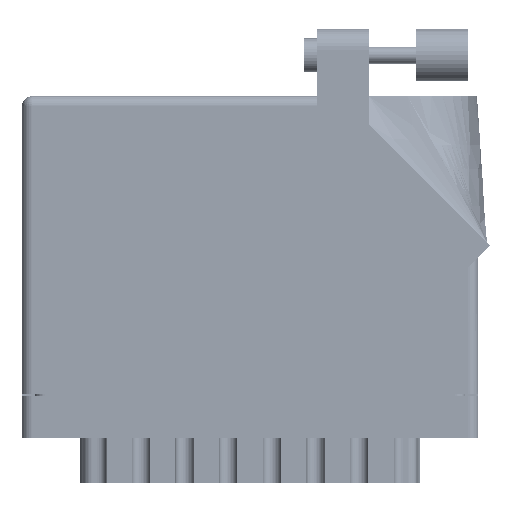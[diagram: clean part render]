
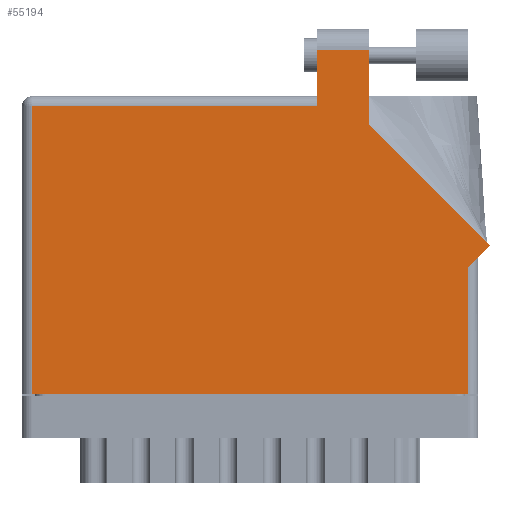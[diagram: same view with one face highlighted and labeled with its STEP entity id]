
A CAD part, front view. The second image highlights one B-rep face of the part: STEP entity #55194.
In plain terms, the highlighted face is planar.
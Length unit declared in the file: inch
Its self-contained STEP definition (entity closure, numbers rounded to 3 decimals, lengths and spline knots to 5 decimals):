
#117 = VECTOR ( 'NONE', #33223, 39.37008 ) ;
#1167 = VERTEX_POINT ( 'NONE', #13531 ) ;
#1967 = LINE ( 'NONE', #8694, #117 ) ;
#3951 = ORIENTED_EDGE ( 'NONE', *, *, #8646, .T. ) ;
#4940 = EDGE_CURVE ( 'NONE', #1167, #25497, #57573, .T. ) ;
#6909 = PLANE ( 'NONE',  #57899 ) ;
#6983 = CARTESIAN_POINT ( 'NONE',  ( 0.062, 1.713, 0. ) ) ;
#8646 = EDGE_CURVE ( 'NONE', #9495, #41288, #15543, .T. ) ;
#8694 = CARTESIAN_POINT ( 'NONE',  ( 1.758, 1.775, 0. ) ) ;
#9495 = VERTEX_POINT ( 'NONE', #6983 ) ;
#10951 = LINE ( 'NONE', #35171, #68198 ) ;
#11305 = ORIENTED_EDGE ( 'NONE', *, *, #34914, .T. ) ;
#13531 = CARTESIAN_POINT ( 'NONE',  ( 2.78871, 0.88571, 0. ) ) ;
#13729 = VECTOR ( 'NONE', #26356, 39.37008 ) ;
#13963 = EDGE_CURVE ( 'NONE', #33533, #1167, #19440, .T. ) ;
#14648 = CARTESIAN_POINT ( 'NONE',  ( 2.656, 0.815, 0. ) ) ;
#15543 = LINE ( 'NONE', #58192, #41485 ) ;
#16351 = DIRECTION ( 'NONE',  ( 0.707, 0.707, 0. ) ) ;
#17807 = DIRECTION ( 'NONE',  ( 1., 0., 0. ) ) ;
#18433 = CARTESIAN_POINT ( 'NONE',  ( 0., 1.713, 0. ) ) ;
#19440 = LINE ( 'NONE', #59026, #32470 ) ;
#19483 = CARTESIAN_POINT ( 'NONE',  ( 0., 1.775, 0. ) ) ;
#21790 = DIRECTION ( 'NONE',  ( 0., 1., 0. ) ) ;
#23983 = VECTOR ( 'NONE', #42228, 39.37008 ) ;
#25497 = VERTEX_POINT ( 'NONE', #66298 ) ;
#26232 = FACE_OUTER_BOUND ( 'NONE', #36542, .T. ) ;
#26356 = DIRECTION ( 'NONE',  ( 0., 1., 0. ) ) ;
#26746 = LINE ( 'NONE', #14648, #13729 ) ;
#29104 = CARTESIAN_POINT ( 'NONE',  ( 1.758, 1.713, 0. ) ) ;
#29597 = EDGE_CURVE ( 'NONE', #49752, #9495, #55372, .T. ) ;
#30723 = LINE ( 'NONE', #57432, #52042 ) ;
#31455 = CARTESIAN_POINT ( 'NONE',  ( 2.656, 0.753, 0. ) ) ;
#31815 = ORIENTED_EDGE ( 'NONE', *, *, #45320, .T. ) ;
#32470 = VECTOR ( 'NONE', #16351, 39.37008 ) ;
#32636 = VECTOR ( 'NONE', #74051, 39.37008 ) ;
#33223 = DIRECTION ( 'NONE',  ( 0., -1., 0. ) ) ;
#33486 = LINE ( 'NONE', #73520, #64881 ) ;
#33533 = VERTEX_POINT ( 'NONE', #31455 ) ;
#34914 = EDGE_CURVE ( 'NONE', #44248, #49752, #1967, .T. ) ;
#35171 = CARTESIAN_POINT ( 'NONE',  ( 0., 0., 0. ) ) ;
#36542 = EDGE_LOOP ( 'NONE', ( #62070, #53210, #11305, #51269, #3951, #51979, #31815, #52541, #62905 ) ) ;
#39656 = EDGE_CURVE ( 'NONE', #41288, #51704, #10951, .T. ) ;
#40179 = CARTESIAN_POINT ( 'NONE',  ( 1.758, 2.05, 0. ) ) ;
#40978 = DIRECTION ( 'NONE',  ( 0., 0., -1. ) ) ;
#41288 = VERTEX_POINT ( 'NONE', #68740 ) ;
#41485 = VECTOR ( 'NONE', #70073, 39.37008 ) ;
#42228 = DIRECTION ( 'NONE',  ( -1., 0., 0. ) ) ;
#44248 = VERTEX_POINT ( 'NONE', #40179 ) ;
#45320 = EDGE_CURVE ( 'NONE', #51704, #33533, #26746, .T. ) ;
#48460 = DIRECTION ( 'NONE',  ( -1., 0., 0. ) ) ;
#49752 = VERTEX_POINT ( 'NONE', #29104 ) ;
#51269 = ORIENTED_EDGE ( 'NONE', *, *, #29597, .T. ) ;
#51704 = VERTEX_POINT ( 'NONE', #68649 ) ;
#51979 = ORIENTED_EDGE ( 'NONE', *, *, #39656, .T. ) ;
#52042 = VECTOR ( 'NONE', #21790, 39.37008 ) ;
#52541 = ORIENTED_EDGE ( 'NONE', *, *, #13963, .T. ) ;
#53210 = ORIENTED_EDGE ( 'NONE', *, *, #56147, .T. ) ;
#55194 = ADVANCED_FACE ( 'NONE', ( #26232 ), #6909, .F. ) ;
#55372 = LINE ( 'NONE', #18433, #23983 ) ;
#55384 = EDGE_CURVE ( 'NONE', #25497, #64626, #30723, .T. ) ;
#55978 = DIRECTION ( 'NONE',  ( -1., 0., 0. ) ) ;
#56147 = EDGE_CURVE ( 'NONE', #64626, #44248, #33486, .T. ) ;
#57432 = CARTESIAN_POINT ( 'NONE',  ( 2.065, 1.60942, 0. ) ) ;
#57573 = LINE ( 'NONE', #61195, #32636 ) ;
#57899 = AXIS2_PLACEMENT_3D ( 'NONE', #19483, #40978, #48460 ) ;
#58192 = CARTESIAN_POINT ( 'NONE',  ( 0.062, 0., 0. ) ) ;
#59026 = CARTESIAN_POINT ( 'NONE',  ( 2.718, 0.815, 0. ) ) ;
#60924 = CARTESIAN_POINT ( 'NONE',  ( 2.065, 2.05, 0. ) ) ;
#61195 = CARTESIAN_POINT ( 'NONE',  ( 2.78871, 0.88571, 0. ) ) ;
#62070 = ORIENTED_EDGE ( 'NONE', *, *, #55384, .T. ) ;
#62905 = ORIENTED_EDGE ( 'NONE', *, *, #4940, .T. ) ;
#64626 = VERTEX_POINT ( 'NONE', #60924 ) ;
#64881 = VECTOR ( 'NONE', #55978, 39.37008 ) ;
#66298 = CARTESIAN_POINT ( 'NONE',  ( 2.065, 1.60942, 0. ) ) ;
#68198 = VECTOR ( 'NONE', #17807, 39.37008 ) ;
#68649 = CARTESIAN_POINT ( 'NONE',  ( 2.656, 0., 0. ) ) ;
#68740 = CARTESIAN_POINT ( 'NONE',  ( 0.062, 0., 0. ) ) ;
#70073 = DIRECTION ( 'NONE',  ( 0., -1., 0. ) ) ;
#73520 = CARTESIAN_POINT ( 'NONE',  ( 1.758, 2.05, 0. ) ) ;
#74051 = DIRECTION ( 'NONE',  ( -0.707, 0.707, 0. ) ) ;
